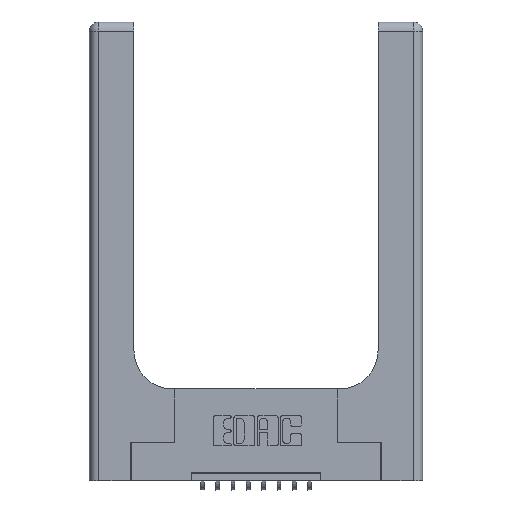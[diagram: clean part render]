
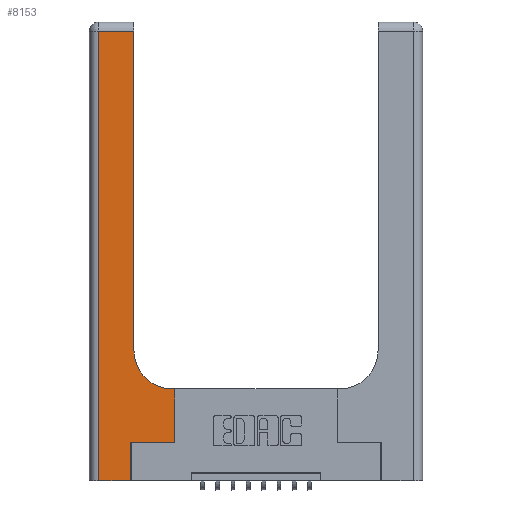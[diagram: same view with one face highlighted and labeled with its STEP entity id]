
A CAD part, top view. The second image highlights one B-rep face of the part: STEP entity #8153.
In plain terms, the highlighted planar face has unit normal (0, 0, 1).
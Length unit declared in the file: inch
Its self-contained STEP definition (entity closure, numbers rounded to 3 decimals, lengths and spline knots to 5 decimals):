
#322 = VERTEX_POINT ( 'NONE', #15616 ) ;
#487 = VECTOR ( 'NONE', #12010, 39.37008 ) ;
#597 = DIRECTION ( 'NONE',  ( 0., 0., -1. ) ) ;
#651 = PLANE ( 'NONE',  #6464 ) ;
#706 = CARTESIAN_POINT ( 'NONE',  ( 0.06, 2.94, 0.37 ) ) ;
#1288 = ORIENTED_EDGE ( 'NONE', *, *, #10179, .T. ) ;
#1325 = CARTESIAN_POINT ( 'NONE',  ( 0.5585, 0.25, 0.37 ) ) ;
#1385 = CARTESIAN_POINT ( 'NONE',  ( 0.5415, 0.85, 0.37 ) ) ;
#1726 = EDGE_LOOP ( 'NONE', ( #1288, #15231, #15811, #2707, #10681, #3974, #4614, #12332, #4521 ) ) ;
#1946 = VECTOR ( 'NONE', #13633, 39.37008 ) ;
#2309 = EDGE_CURVE ( 'NONE', #4045, #322, #9502, .T. ) ;
#2687 = VECTOR ( 'NONE', #9703, 39.37008 ) ;
#2707 = ORIENTED_EDGE ( 'NONE', *, *, #12962, .T. ) ;
#2720 = DIRECTION ( 'NONE',  ( 0., 0., -1. ) ) ;
#2724 = AXIS2_PLACEMENT_3D ( 'NONE', #1385, #2720, #11211 ) ;
#3159 = CARTESIAN_POINT ( 'NONE',  ( 0., 3., 0.37 ) ) ;
#3929 = EDGE_CURVE ( 'NONE', #10553, #10174, #7099, .T. ) ;
#3974 = ORIENTED_EDGE ( 'NONE', *, *, #6767, .T. ) ;
#4045 = VERTEX_POINT ( 'NONE', #14688 ) ;
#4051 = CARTESIAN_POINT ( 'NONE',  ( 0.06, 0., 0.37 ) ) ;
#4397 = EDGE_CURVE ( 'NONE', #10174, #6313, #8991, .T. ) ;
#4521 = ORIENTED_EDGE ( 'NONE', *, *, #15883, .T. ) ;
#4603 = VECTOR ( 'NONE', #13161, 39.37008 ) ;
#4614 = ORIENTED_EDGE ( 'NONE', *, *, #3929, .T. ) ;
#4702 = LINE ( 'NONE', #10571, #487 ) ;
#4891 = CARTESIAN_POINT ( 'NONE',  ( 0.269, 0.25, 0.37 ) ) ;
#5178 = VECTOR ( 'NONE', #5232, 39.37008 ) ;
#5232 = DIRECTION ( 'NONE',  ( -1., 0., 0. ) ) ;
#5732 = DIRECTION ( 'NONE',  ( -1., 0., 0. ) ) ;
#5740 = DIRECTION ( 'NONE',  ( 1., 0., 0. ) ) ;
#5769 = LINE ( 'NONE', #11260, #1946 ) ;
#5901 = CARTESIAN_POINT ( 'NONE',  ( 0., 0., 0.37 ) ) ;
#6255 = CIRCLE ( 'NONE', #2724, 0.25 ) ;
#6286 = LINE ( 'NONE', #4891, #14086 ) ;
#6313 = VERTEX_POINT ( 'NONE', #10308 ) ;
#6464 = AXIS2_PLACEMENT_3D ( 'NONE', #3159, #597, #5732 ) ;
#6767 = EDGE_CURVE ( 'NONE', #322, #10553, #6286, .T. ) ;
#7099 = LINE ( 'NONE', #1325, #2687 ) ;
#7190 = FACE_OUTER_BOUND ( 'NONE', #1726, .T. ) ;
#7418 = VECTOR ( 'NONE', #12416, 39.37008 ) ;
#7940 = CARTESIAN_POINT ( 'NONE',  ( 0.5585, 0.6, 0.37 ) ) ;
#8153 = ADVANCED_FACE ( 'NONE', ( #7190 ), #651, .F. ) ;
#8173 = VERTEX_POINT ( 'NONE', #706 ) ;
#8671 = CARTESIAN_POINT ( 'NONE',  ( 0.2915, 0.85, 0.37 ) ) ;
#8726 = CARTESIAN_POINT ( 'NONE',  ( 0.5585, 0.25, 0.37 ) ) ;
#8991 = LINE ( 'NONE', #10128, #5178 ) ;
#9004 = LINE ( 'NONE', #5901, #12040 ) ;
#9502 = LINE ( 'NONE', #14868, #7418 ) ;
#9703 = DIRECTION ( 'NONE',  ( 0., 1., 0. ) ) ;
#9823 = VERTEX_POINT ( 'NONE', #13697 ) ;
#10128 = CARTESIAN_POINT ( 'NONE',  ( 0.2915, 0.6, 0.37 ) ) ;
#10174 = VERTEX_POINT ( 'NONE', #7940 ) ;
#10179 = EDGE_CURVE ( 'NONE', #13598, #9823, #4702, .T. ) ;
#10308 = CARTESIAN_POINT ( 'NONE',  ( 0.5415, 0.6, 0.37 ) ) ;
#10553 = VERTEX_POINT ( 'NONE', #8726 ) ;
#10571 = CARTESIAN_POINT ( 'NONE',  ( 0.2915, 3., 0.37 ) ) ;
#10681 = ORIENTED_EDGE ( 'NONE', *, *, #2309, .T. ) ;
#11211 = DIRECTION ( 'NONE',  ( 1., 0., 0. ) ) ;
#11260 = CARTESIAN_POINT ( 'NONE',  ( 0.06, 3., 0.37 ) ) ;
#12010 = DIRECTION ( 'NONE',  ( 0., 1., 0. ) ) ;
#12040 = VECTOR ( 'NONE', #5740, 39.37008 ) ;
#12122 = EDGE_CURVE ( 'NONE', #8173, #13307, #5769, .T. ) ;
#12332 = ORIENTED_EDGE ( 'NONE', *, *, #4397, .T. ) ;
#12416 = DIRECTION ( 'NONE',  ( 0., 1., 0. ) ) ;
#12962 = EDGE_CURVE ( 'NONE', #13307, #4045, #9004, .T. ) ;
#13011 = LINE ( 'NONE', #13210, #4603 ) ;
#13081 = EDGE_CURVE ( 'NONE', #9823, #8173, #13011, .T. ) ;
#13161 = DIRECTION ( 'NONE',  ( -1., 0., 0. ) ) ;
#13210 = CARTESIAN_POINT ( 'NONE',  ( 0., 2.94, 0.37 ) ) ;
#13307 = VERTEX_POINT ( 'NONE', #4051 ) ;
#13428 = DIRECTION ( 'NONE',  ( 1., 0., 0. ) ) ;
#13598 = VERTEX_POINT ( 'NONE', #8671 ) ;
#13633 = DIRECTION ( 'NONE',  ( 0., -1., 0. ) ) ;
#13697 = CARTESIAN_POINT ( 'NONE',  ( 0.2915, 2.94, 0.37 ) ) ;
#14086 = VECTOR ( 'NONE', #13428, 39.37008 ) ;
#14688 = CARTESIAN_POINT ( 'NONE',  ( 0.269, 0., 0.37 ) ) ;
#14868 = CARTESIAN_POINT ( 'NONE',  ( 0.269, 0., 0.37 ) ) ;
#15231 = ORIENTED_EDGE ( 'NONE', *, *, #13081, .T. ) ;
#15616 = CARTESIAN_POINT ( 'NONE',  ( 0.269, 0.25, 0.37 ) ) ;
#15811 = ORIENTED_EDGE ( 'NONE', *, *, #12122, .T. ) ;
#15883 = EDGE_CURVE ( 'NONE', #6313, #13598, #6255, .T. ) ;
